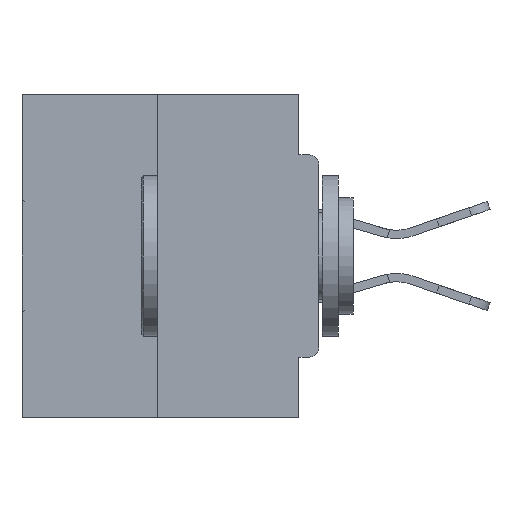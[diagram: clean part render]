
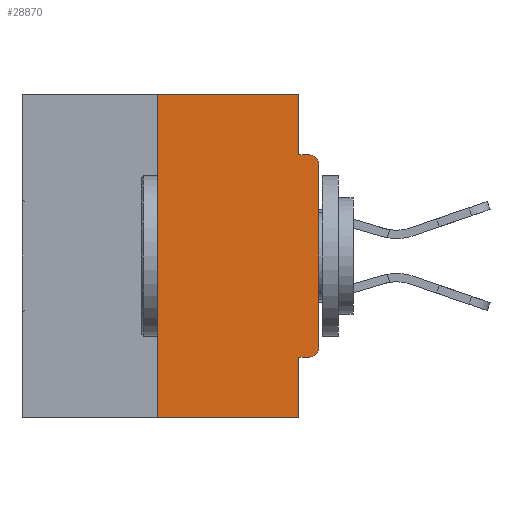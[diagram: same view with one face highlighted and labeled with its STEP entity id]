
A CAD part, left-side view. The second image highlights one B-rep face of the part: STEP entity #28870.
In plain terms, the highlighted planar face has unit normal (-1, 0, 0).
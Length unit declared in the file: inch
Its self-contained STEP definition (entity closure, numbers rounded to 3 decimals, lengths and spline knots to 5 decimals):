
#143 = CARTESIAN_POINT ( 'NONE',  ( 0., 0.25, 0. ) ) ;
#156 = LINE ( 'NONE', #7074, #5295 ) ;
#805 = LINE ( 'NONE', #10357, #8906 ) ;
#997 = FACE_OUTER_BOUND ( 'NONE', #35756, .T. ) ;
#1268 = CARTESIAN_POINT ( 'NONE',  ( 0., 0.25, -0.5 ) ) ;
#1317 = VERTEX_POINT ( 'NONE', #26366 ) ;
#2212 = EDGE_CURVE ( 'NONE', #14339, #23832, #8309, .T. ) ;
#2982 = DIRECTION ( 'NONE',  ( -1., 0., 0. ) ) ;
#3008 = DIRECTION ( 'NONE',  ( 0., 0., -1. ) ) ;
#3036 = VERTEX_POINT ( 'NONE', #27307 ) ;
#4363 = VECTOR ( 'NONE', #35051, 39.37008 ) ;
#4651 = EDGE_CURVE ( 'NONE', #28507, #3036, #34184, .T. ) ;
#5086 = DIRECTION ( 'NONE',  ( 0., 0., -1. ) ) ;
#5295 = VECTOR ( 'NONE', #16682, 39.37008 ) ;
#5763 = ORIENTED_EDGE ( 'NONE', *, *, #17048, .T. ) ;
#6461 = CIRCLE ( 'NONE', #26238, 0.015 ) ;
#6682 = CARTESIAN_POINT ( 'NONE',  ( 0., 0.015, -0.1085 ) ) ;
#7074 = CARTESIAN_POINT ( 'NONE',  ( 0., 0.25, 0. ) ) ;
#7325 = DIRECTION ( 'NONE',  ( 1., 0., 0. ) ) ;
#8309 = LINE ( 'NONE', #12042, #18439 ) ;
#8709 = LINE ( 'NONE', #21559, #36384 ) ;
#8906 = VECTOR ( 'NONE', #40180, 39.37008 ) ;
#9440 = VERTEX_POINT ( 'NONE', #1268 ) ;
#10357 = CARTESIAN_POINT ( 'NONE',  ( 0., 0., 0. ) ) ;
#10408 = DIRECTION ( 'NONE',  ( 0., 0., -1. ) ) ;
#10692 = ORIENTED_EDGE ( 'NONE', *, *, #17831, .F. ) ;
#11957 = CARTESIAN_POINT ( 'NONE',  ( 0., 0.031, 0. ) ) ;
#12042 = CARTESIAN_POINT ( 'NONE',  ( 0., 0.46, 0. ) ) ;
#12234 = CARTESIAN_POINT ( 'NONE',  ( 0., 0., -0.4065 ) ) ;
#13434 = EDGE_CURVE ( 'NONE', #28229, #28507, #805, .T. ) ;
#13616 = PLANE ( 'NONE',  #39709 ) ;
#14000 = ORIENTED_EDGE ( 'NONE', *, *, #24775, .F. ) ;
#14339 = VERTEX_POINT ( 'NONE', #143 ) ;
#14393 = VECTOR ( 'NONE', #36011, 39.37008 ) ;
#15489 = CARTESIAN_POINT ( 'NONE',  ( 0., 0., -0.3915 ) ) ;
#15701 = ORIENTED_EDGE ( 'NONE', *, *, #18822, .F. ) ;
#15924 = AXIS2_PLACEMENT_3D ( 'NONE', #6682, #2982, #22655 ) ;
#15929 = ORIENTED_EDGE ( 'NONE', *, *, #2212, .F. ) ;
#15967 = VECTOR ( 'NONE', #5086, 39.37008 ) ;
#16682 = DIRECTION ( 'NONE',  ( 0., 0., 1. ) ) ;
#17048 = EDGE_CURVE ( 'NONE', #1317, #28229, #6461, .T. ) ;
#17357 = ORIENTED_EDGE ( 'NONE', *, *, #37473, .F. ) ;
#17831 = EDGE_CURVE ( 'NONE', #33082, #3036, #31452, .T. ) ;
#18439 = VECTOR ( 'NONE', #21525, 39.37008 ) ;
#18527 = VERTEX_POINT ( 'NONE', #18573 ) ;
#18573 = CARTESIAN_POINT ( 'NONE',  ( 0., 0.031, -0.4065 ) ) ;
#18623 = CARTESIAN_POINT ( 'NONE',  ( 0., 0.015, -0.3915 ) ) ;
#18822 = EDGE_CURVE ( 'NONE', #9440, #14339, #156, .T. ) ;
#20121 = VECTOR ( 'NONE', #30161, 39.37008 ) ;
#21182 = VERTEX_POINT ( 'NONE', #41042 ) ;
#21525 = DIRECTION ( 'NONE',  ( 0., -1., 0. ) ) ;
#21559 = CARTESIAN_POINT ( 'NONE',  ( 0., 0.46, -0.5 ) ) ;
#22655 = DIRECTION ( 'NONE',  ( 0., 0., -1. ) ) ;
#23832 = VERTEX_POINT ( 'NONE', #11957 ) ;
#24775 = EDGE_CURVE ( 'NONE', #1317, #18527, #37612, .T. ) ;
#25796 = LINE ( 'NONE', #31386, #15967 ) ;
#26238 = AXIS2_PLACEMENT_3D ( 'NONE', #18623, #35458, #3008 ) ;
#26366 = CARTESIAN_POINT ( 'NONE',  ( 0., 0.015, -0.4065 ) ) ;
#27307 = CARTESIAN_POINT ( 'NONE',  ( 0., 0.015, -0.0935 ) ) ;
#27326 = LINE ( 'NONE', #36570, #14393 ) ;
#27562 = EDGE_CURVE ( 'NONE', #9440, #21182, #8709, .T. ) ;
#28229 = VERTEX_POINT ( 'NONE', #15489 ) ;
#28507 = VERTEX_POINT ( 'NONE', #37321 ) ;
#28870 = ADVANCED_FACE ( 'NONE', ( #997 ), #13616, .F. ) ;
#29566 = ORIENTED_EDGE ( 'NONE', *, *, #13434, .T. ) ;
#30161 = DIRECTION ( 'NONE',  ( 0., -1., 0. ) ) ;
#31386 = CARTESIAN_POINT ( 'NONE',  ( 0., 0.031, 0. ) ) ;
#31452 = LINE ( 'NONE', #35800, #20121 ) ;
#31525 = EDGE_CURVE ( 'NONE', #23832, #33082, #25796, .T. ) ;
#33082 = VERTEX_POINT ( 'NONE', #40778 ) ;
#34184 = CIRCLE ( 'NONE', #15924, 0.015 ) ;
#35038 = DIRECTION ( 'NONE',  ( 0., -1., 0. ) ) ;
#35040 = ORIENTED_EDGE ( 'NONE', *, *, #27562, .T. ) ;
#35051 = DIRECTION ( 'NONE',  ( 0., 1., 0. ) ) ;
#35458 = DIRECTION ( 'NONE',  ( -1., 0., 0. ) ) ;
#35756 = EDGE_LOOP ( 'NONE', ( #15929, #15701, #35040, #17357, #14000, #5763, #29566, #40724, #10692, #40346 ) ) ;
#35800 = CARTESIAN_POINT ( 'NONE',  ( 0., 0., -0.0935 ) ) ;
#36011 = DIRECTION ( 'NONE',  ( 0., 0., -1. ) ) ;
#36360 = CARTESIAN_POINT ( 'NONE',  ( 0., 0.46, 0. ) ) ;
#36384 = VECTOR ( 'NONE', #35038, 39.37008 ) ;
#36570 = CARTESIAN_POINT ( 'NONE',  ( 0., 0.031, -0.5 ) ) ;
#37321 = CARTESIAN_POINT ( 'NONE',  ( 0., 0., -0.1085 ) ) ;
#37473 = EDGE_CURVE ( 'NONE', #18527, #21182, #27326, .T. ) ;
#37612 = LINE ( 'NONE', #12234, #4363 ) ;
#39709 = AXIS2_PLACEMENT_3D ( 'NONE', #36360, #7325, #10408 ) ;
#40180 = DIRECTION ( 'NONE',  ( 0., 0., 1. ) ) ;
#40346 = ORIENTED_EDGE ( 'NONE', *, *, #31525, .F. ) ;
#40724 = ORIENTED_EDGE ( 'NONE', *, *, #4651, .T. ) ;
#40778 = CARTESIAN_POINT ( 'NONE',  ( 0., 0.031, -0.0935 ) ) ;
#41042 = CARTESIAN_POINT ( 'NONE',  ( 0., 0.031, -0.5 ) ) ;
